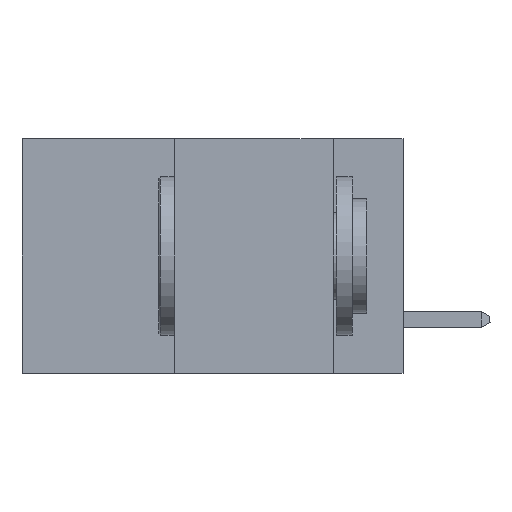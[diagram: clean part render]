
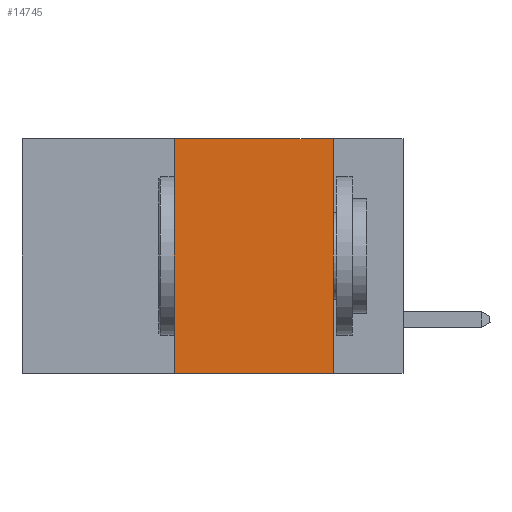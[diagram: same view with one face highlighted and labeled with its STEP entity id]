
A CAD part, left-side view. The second image highlights one B-rep face of the part: STEP entity #14745.
In plain terms, the highlighted planar face has unit normal (-1, 0, 0).
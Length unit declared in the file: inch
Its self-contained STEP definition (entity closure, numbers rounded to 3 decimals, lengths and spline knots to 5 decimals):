
#592 = CARTESIAN_POINT ( 'NONE',  ( 0., 0.11, -0.37 ) ) ;
#1353 = DIRECTION ( 'NONE',  ( 0., -1., 0. ) ) ;
#1540 = ORIENTED_EDGE ( 'NONE', *, *, #5230, .F. ) ;
#2308 = DIRECTION ( 'NONE',  ( 0., -1., 0. ) ) ;
#4576 = CARTESIAN_POINT ( 'NONE',  ( 0., 0.36, -0.37 ) ) ;
#4683 = DIRECTION ( 'NONE',  ( 0., 0., -1. ) ) ;
#4832 = CARTESIAN_POINT ( 'NONE',  ( 0., 0.6, 0. ) ) ;
#5230 = EDGE_CURVE ( 'NONE', #6397, #23033, #21755, .T. ) ;
#5712 = VECTOR ( 'NONE', #2308, 39.37008 ) ;
#6244 = CARTESIAN_POINT ( 'NONE',  ( 0., 0.6, 0. ) ) ;
#6397 = VERTEX_POINT ( 'NONE', #4576 ) ;
#6483 = CARTESIAN_POINT ( 'NONE',  ( 0., 0.36, 0. ) ) ;
#6710 = DIRECTION ( 'NONE',  ( 1., 0., 0. ) ) ;
#7558 = LINE ( 'NONE', #6244, #5712 ) ;
#7721 = AXIS2_PLACEMENT_3D ( 'NONE', #4832, #6710, #4683 ) ;
#7736 = CARTESIAN_POINT ( 'NONE',  ( 0., 0.36, 0. ) ) ;
#7909 = EDGE_CURVE ( 'NONE', #6397, #12743, #16880, .T. ) ;
#8068 = VERTEX_POINT ( 'NONE', #22041 ) ;
#8620 = VECTOR ( 'NONE', #15215, 39.37008 ) ;
#9136 = ORIENTED_EDGE ( 'NONE', *, *, #23571, .F. ) ;
#9760 = EDGE_CURVE ( 'NONE', #23033, #8068, #7558, .T. ) ;
#9773 = FACE_OUTER_BOUND ( 'NONE', #13309, .T. ) ;
#9884 = LINE ( 'NONE', #17132, #8620 ) ;
#11133 = ORIENTED_EDGE ( 'NONE', *, *, #9760, .F. ) ;
#12182 = DIRECTION ( 'NONE',  ( 0., 0., 1. ) ) ;
#12743 = VERTEX_POINT ( 'NONE', #592 ) ;
#13309 = EDGE_LOOP ( 'NONE', ( #9136, #11133, #1540, #18003 ) ) ;
#14745 = ADVANCED_FACE ( 'NONE', ( #9773 ), #18301, .F. ) ;
#14847 = VECTOR ( 'NONE', #12182, 39.37008 ) ;
#15215 = DIRECTION ( 'NONE',  ( 0., 0., -1. ) ) ;
#16880 = LINE ( 'NONE', #24485, #22884 ) ;
#17132 = CARTESIAN_POINT ( 'NONE',  ( 0., 0.11, 0. ) ) ;
#18003 = ORIENTED_EDGE ( 'NONE', *, *, #7909, .T. ) ;
#18301 = PLANE ( 'NONE',  #7721 ) ;
#21755 = LINE ( 'NONE', #6483, #14847 ) ;
#22041 = CARTESIAN_POINT ( 'NONE',  ( 0., 0.11, 0. ) ) ;
#22884 = VECTOR ( 'NONE', #1353, 39.37008 ) ;
#23033 = VERTEX_POINT ( 'NONE', #7736 ) ;
#23571 = EDGE_CURVE ( 'NONE', #8068, #12743, #9884, .T. ) ;
#24485 = CARTESIAN_POINT ( 'NONE',  ( 0., 0.6, -0.37 ) ) ;
